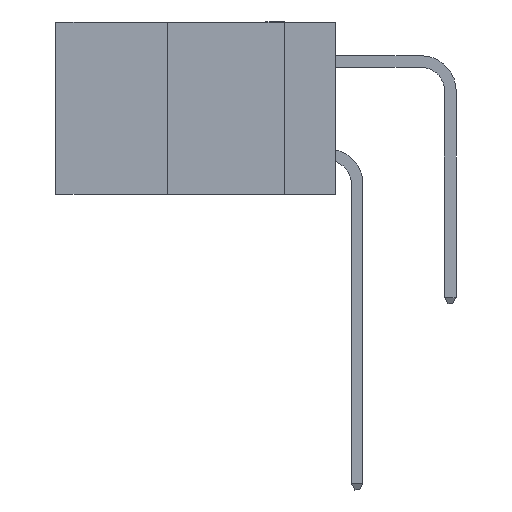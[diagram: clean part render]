
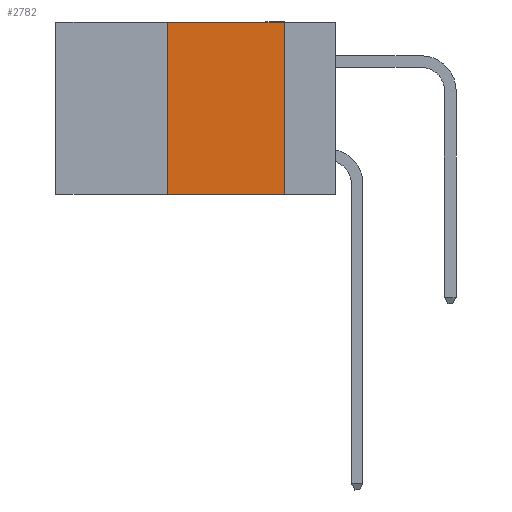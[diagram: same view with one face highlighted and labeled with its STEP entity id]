
A CAD part, left-side view. The second image highlights one B-rep face of the part: STEP entity #2782.
In plain terms, the highlighted planar face has unit normal (-1, 0, 0).
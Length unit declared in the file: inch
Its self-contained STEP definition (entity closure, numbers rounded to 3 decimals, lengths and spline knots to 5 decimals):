
#161 = DIRECTION ( 'NONE',  ( 0., -1., 0. ) ) ;
#723 = CARTESIAN_POINT ( 'NONE',  ( 0., 0.6, 0. ) ) ;
#1313 = AXIS2_PLACEMENT_3D ( 'NONE', #723, #1545, #10722 ) ;
#1545 = DIRECTION ( 'NONE',  ( 1., 0., 0. ) ) ;
#1962 = VERTEX_POINT ( 'NONE', #5734 ) ;
#2782 = ADVANCED_FACE ( 'NONE', ( #9703 ), #7115, .F. ) ;
#3145 = EDGE_CURVE ( 'NONE', #6254, #10412, #10534, .T. ) ;
#3278 = VECTOR ( 'NONE', #9754, 39.37008 ) ;
#3293 = EDGE_CURVE ( 'NONE', #6254, #10690, #4452, .T. ) ;
#3560 = CARTESIAN_POINT ( 'NONE',  ( 0., 0.6, -0.37 ) ) ;
#3814 = ORIENTED_EDGE ( 'NONE', *, *, #9143, .F. ) ;
#3911 = LINE ( 'NONE', #10352, #10538 ) ;
#4097 = LINE ( 'NONE', #9582, #3278 ) ;
#4452 = LINE ( 'NONE', #3560, #8463 ) ;
#4924 = DIRECTION ( 'NONE',  ( 0., 0., -1. ) ) ;
#5205 = CARTESIAN_POINT ( 'NONE',  ( 0., 0.36, 0. ) ) ;
#5734 = CARTESIAN_POINT ( 'NONE',  ( 0., 0.11, 0. ) ) ;
#6254 = VERTEX_POINT ( 'NONE', #6778 ) ;
#6531 = EDGE_LOOP ( 'NONE', ( #3814, #6564, #10397, #7244 ) ) ;
#6564 = ORIENTED_EDGE ( 'NONE', *, *, #7737, .F. ) ;
#6778 = CARTESIAN_POINT ( 'NONE',  ( 0., 0.36, -0.37 ) ) ;
#6805 = CARTESIAN_POINT ( 'NONE',  ( 0., 0.11, -0.37 ) ) ;
#7115 = PLANE ( 'NONE',  #1313 ) ;
#7244 = ORIENTED_EDGE ( 'NONE', *, *, #3293, .T. ) ;
#7737 = EDGE_CURVE ( 'NONE', #10412, #1962, #4097, .T. ) ;
#7973 = DIRECTION ( 'NONE',  ( 0., 0., 1. ) ) ;
#8463 = VECTOR ( 'NONE', #161, 39.37008 ) ;
#9143 = EDGE_CURVE ( 'NONE', #1962, #10690, #3911, .T. ) ;
#9460 = VECTOR ( 'NONE', #7973, 39.37008 ) ;
#9582 = CARTESIAN_POINT ( 'NONE',  ( 0., 0.6, 0. ) ) ;
#9703 = FACE_OUTER_BOUND ( 'NONE', #6531, .T. ) ;
#9754 = DIRECTION ( 'NONE',  ( 0., -1., 0. ) ) ;
#9864 = CARTESIAN_POINT ( 'NONE',  ( 0., 0.36, 0. ) ) ;
#10352 = CARTESIAN_POINT ( 'NONE',  ( 0., 0.11, 0. ) ) ;
#10397 = ORIENTED_EDGE ( 'NONE', *, *, #3145, .F. ) ;
#10412 = VERTEX_POINT ( 'NONE', #5205 ) ;
#10534 = LINE ( 'NONE', #9864, #9460 ) ;
#10538 = VECTOR ( 'NONE', #4924, 39.37008 ) ;
#10690 = VERTEX_POINT ( 'NONE', #6805 ) ;
#10722 = DIRECTION ( 'NONE',  ( 0., 0., -1. ) ) ;
